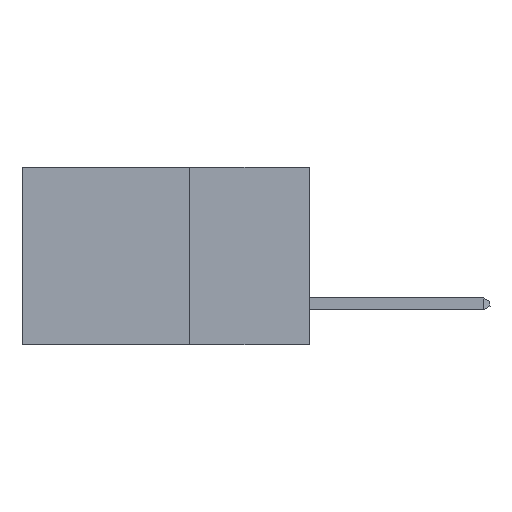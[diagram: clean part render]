
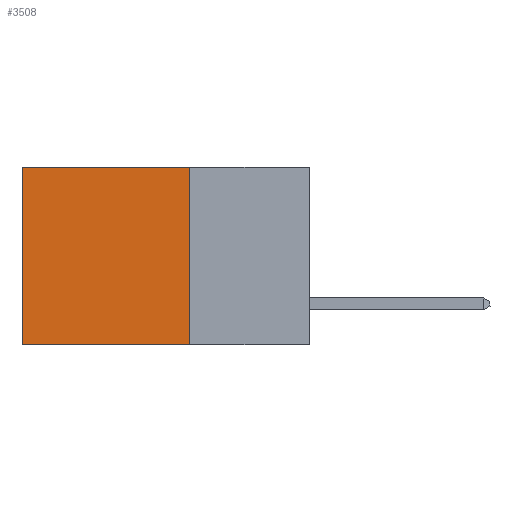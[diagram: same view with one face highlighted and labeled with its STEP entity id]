
A CAD part, left-side view. The second image highlights one B-rep face of the part: STEP entity #3508.
In plain terms, the highlighted planar face has unit normal (-1, 0, 0).
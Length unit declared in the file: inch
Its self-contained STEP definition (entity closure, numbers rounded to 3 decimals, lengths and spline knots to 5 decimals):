
#178 = DIRECTION ( 'NONE',  ( 0., 1., 0. ) ) ;
#254 = CARTESIAN_POINT ( 'NONE',  ( 0.2875, 0.25, -0.37 ) ) ;
#261 = VERTEX_POINT ( 'NONE', #1983 ) ;
#368 = ORIENTED_EDGE ( 'NONE', *, *, #5061, .T. ) ;
#412 = VECTOR ( 'NONE', #8240, 39.37008 ) ;
#718 = ORIENTED_EDGE ( 'NONE', *, *, #7454, .F. ) ;
#953 = AXIS2_PLACEMENT_3D ( 'NONE', #10318, #10130, #10127 ) ;
#1067 = CARTESIAN_POINT ( 'NONE',  ( 0.2875, 0.25, 0. ) ) ;
#1513 = CARTESIAN_POINT ( 'NONE',  ( 0.2875, 0.6, 0. ) ) ;
#1725 = EDGE_CURVE ( 'NONE', #6227, #10005, #5180, .T. ) ;
#1766 = VERTEX_POINT ( 'NONE', #1067 ) ;
#1983 = CARTESIAN_POINT ( 'NONE',  ( 0.2875, 0.6, 0. ) ) ;
#2108 = VECTOR ( 'NONE', #178, 39.37008 ) ;
#3317 = CARTESIAN_POINT ( 'NONE',  ( 0.2875, 0.25, 0. ) ) ;
#3376 = CARTESIAN_POINT ( 'NONE',  ( 0.2875, 0.25, 0. ) ) ;
#3415 = LINE ( 'NONE', #1513, #412 ) ;
#3441 = ORIENTED_EDGE ( 'NONE', *, *, #1725, .F. ) ;
#3508 = ADVANCED_FACE ( 'NONE', ( #4595 ), #10206, .F. ) ;
#4354 = VECTOR ( 'NONE', #10002, 39.37008 ) ;
#4595 = FACE_OUTER_BOUND ( 'NONE', #7452, .T. ) ;
#5061 = EDGE_CURVE ( 'NONE', #1766, #261, #7288, .T. ) ;
#5180 = LINE ( 'NONE', #254, #2108 ) ;
#5307 = EDGE_CURVE ( 'NONE', #261, #10005, #3415, .T. ) ;
#6227 = VERTEX_POINT ( 'NONE', #12127 ) ;
#7288 = LINE ( 'NONE', #3376, #4354 ) ;
#7452 = EDGE_LOOP ( 'NONE', ( #8980, #3441, #718, #368 ) ) ;
#7454 = EDGE_CURVE ( 'NONE', #1766, #6227, #10109, .T. ) ;
#7882 = CARTESIAN_POINT ( 'NONE',  ( 0.2875, 0.6, -0.37 ) ) ;
#8240 = DIRECTION ( 'NONE',  ( 0., 0., -1. ) ) ;
#8980 = ORIENTED_EDGE ( 'NONE', *, *, #5307, .T. ) ;
#10002 = DIRECTION ( 'NONE',  ( 0., 1., 0. ) ) ;
#10005 = VERTEX_POINT ( 'NONE', #7882 ) ;
#10109 = LINE ( 'NONE', #3317, #12633 ) ;
#10127 = DIRECTION ( 'NONE',  ( 0., 0., -1. ) ) ;
#10130 = DIRECTION ( 'NONE',  ( 1., 0., 0. ) ) ;
#10206 = PLANE ( 'NONE',  #953 ) ;
#10318 = CARTESIAN_POINT ( 'NONE',  ( 0.2875, 0.25, 0. ) ) ;
#12127 = CARTESIAN_POINT ( 'NONE',  ( 0.2875, 0.25, -0.37 ) ) ;
#12633 = VECTOR ( 'NONE', #14191, 39.37008 ) ;
#14191 = DIRECTION ( 'NONE',  ( 0., 0., -1. ) ) ;
